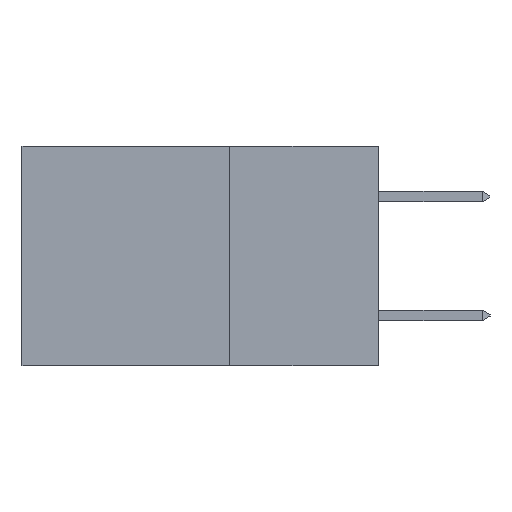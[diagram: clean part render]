
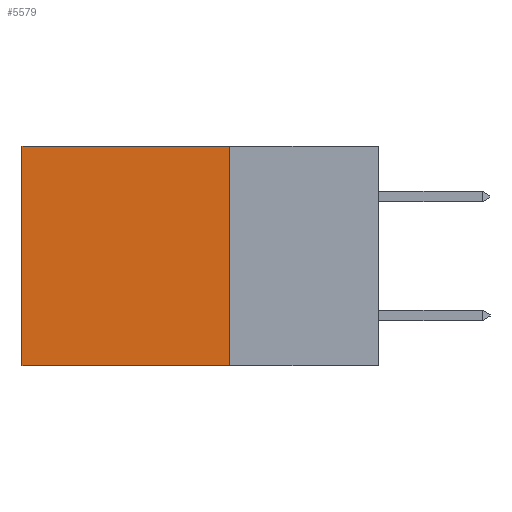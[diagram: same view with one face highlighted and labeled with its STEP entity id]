
A CAD part, left-side view. The second image highlights one B-rep face of the part: STEP entity #5579.
In plain terms, the highlighted planar face has unit normal (-1, 0, 0).
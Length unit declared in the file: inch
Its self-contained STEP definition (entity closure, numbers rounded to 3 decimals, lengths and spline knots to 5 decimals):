
#205 = VERTEX_POINT ( 'NONE', #1843 ) ;
#507 = EDGE_CURVE ( 'NONE', #14796, #205, #3411, .T. ) ;
#962 = DIRECTION ( 'NONE',  ( 0., 1., 0. ) ) ;
#1433 = VERTEX_POINT ( 'NONE', #14604 ) ;
#1843 = CARTESIAN_POINT ( 'NONE',  ( 0.2615, 0.6, -0.37 ) ) ;
#2217 = DIRECTION ( 'NONE',  ( 0., 0., -1. ) ) ;
#2508 = ORIENTED_EDGE ( 'NONE', *, *, #507, .F. ) ;
#3411 = LINE ( 'NONE', #6706, #10462 ) ;
#3604 = ORIENTED_EDGE ( 'NONE', *, *, #10110, .T. ) ;
#3664 = CARTESIAN_POINT ( 'NONE',  ( 0.2615, 0.25, 0. ) ) ;
#3954 = LINE ( 'NONE', #9259, #11003 ) ;
#5212 = VECTOR ( 'NONE', #12177, 39.37008 ) ;
#5579 = ADVANCED_FACE ( 'NONE', ( #16785 ), #17572, .F. ) ;
#6275 = DIRECTION ( 'NONE',  ( 1., 0., 0. ) ) ;
#6706 = CARTESIAN_POINT ( 'NONE',  ( 0.2615, 0.25, -0.37 ) ) ;
#8027 = EDGE_CURVE ( 'NONE', #12824, #205, #3954, .T. ) ;
#8511 = VECTOR ( 'NONE', #17972, 39.37008 ) ;
#8933 = AXIS2_PLACEMENT_3D ( 'NONE', #11941, #6275, #16225 ) ;
#9259 = CARTESIAN_POINT ( 'NONE',  ( 0.2615, 0.6, -0.37 ) ) ;
#9344 = ORIENTED_EDGE ( 'NONE', *, *, #15047, .F. ) ;
#10110 = EDGE_CURVE ( 'NONE', #1433, #12824, #16514, .T. ) ;
#10324 = EDGE_LOOP ( 'NONE', ( #10363, #2508, #9344, #3604 ) ) ;
#10363 = ORIENTED_EDGE ( 'NONE', *, *, #8027, .T. ) ;
#10462 = VECTOR ( 'NONE', #962, 39.37008 ) ;
#11003 = VECTOR ( 'NONE', #2217, 39.37008 ) ;
#11941 = CARTESIAN_POINT ( 'NONE',  ( 0.2615, 0.25, -0.37 ) ) ;
#11992 = CARTESIAN_POINT ( 'NONE',  ( 0.2615, 0.6, 0. ) ) ;
#12177 = DIRECTION ( 'NONE',  ( 0., 1., 0. ) ) ;
#12356 = LINE ( 'NONE', #13736, #8511 ) ;
#12824 = VERTEX_POINT ( 'NONE', #11992 ) ;
#13736 = CARTESIAN_POINT ( 'NONE',  ( 0.2615, 0.25, -0.37 ) ) ;
#14604 = CARTESIAN_POINT ( 'NONE',  ( 0.2615, 0.25, 0. ) ) ;
#14796 = VERTEX_POINT ( 'NONE', #17421 ) ;
#15047 = EDGE_CURVE ( 'NONE', #1433, #14796, #12356, .T. ) ;
#16225 = DIRECTION ( 'NONE',  ( 0., 0., -1. ) ) ;
#16514 = LINE ( 'NONE', #3664, #5212 ) ;
#16785 = FACE_OUTER_BOUND ( 'NONE', #10324, .T. ) ;
#17421 = CARTESIAN_POINT ( 'NONE',  ( 0.2615, 0.25, -0.37 ) ) ;
#17572 = PLANE ( 'NONE',  #8933 ) ;
#17972 = DIRECTION ( 'NONE',  ( 0., 0., -1. ) ) ;
